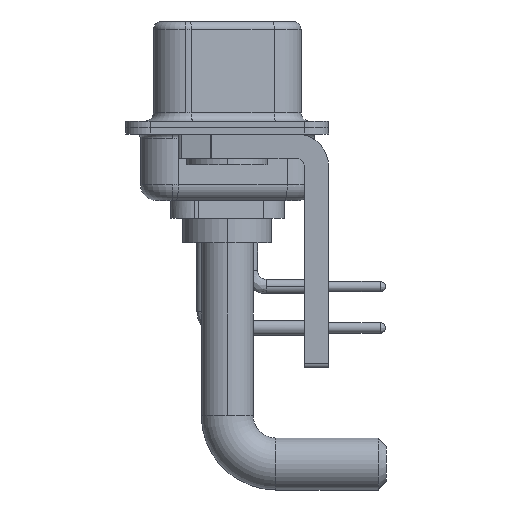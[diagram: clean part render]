
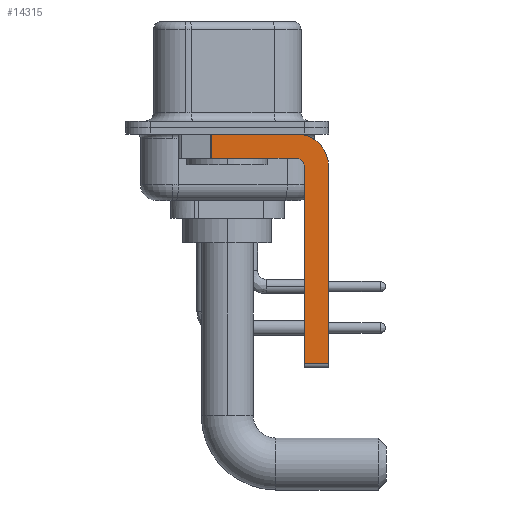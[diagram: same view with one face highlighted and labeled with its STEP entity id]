
A CAD part, left-side view. The second image highlights one B-rep face of the part: STEP entity #14315.
In plain terms, the highlighted planar face has unit normal (-1, 0, 0).
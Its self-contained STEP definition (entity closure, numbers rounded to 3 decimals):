
#179 = VERTEX_POINT ( 'NONE', #17089 ) ;
#199 = CARTESIAN_POINT ( 'NONE',  ( -2.9, -6.25, -2.4 ) ) ;
#289 = PLANE ( 'NONE',  #7650 ) ;
#544 = DIRECTION ( 'NONE',  ( 1., 0., 0. ) ) ;
#666 = DIRECTION ( 'NONE',  ( 0., 0., -1. ) ) ;
#1107 = ORIENTED_EDGE ( 'NONE', *, *, #8212, .T. ) ;
#1223 = ORIENTED_EDGE ( 'NONE', *, *, #15616, .F. ) ;
#1299 = CARTESIAN_POINT ( 'NONE',  ( -2.9, -4.25, -0.4 ) ) ;
#1308 = ORIENTED_EDGE ( 'NONE', *, *, #18619, .F. ) ;
#1354 = VERTEX_POINT ( 'NONE', #23526 ) ;
#1426 = CARTESIAN_POINT ( 'NONE',  ( -2.9, -4.75, -14.8 ) ) ;
#1661 = LINE ( 'NONE', #19299, #11949 ) ;
#1909 = VECTOR ( 'NONE', #19220, 1000. ) ;
#2603 = LINE ( 'NONE', #199, #24019 ) ;
#2900 = VERTEX_POINT ( 'NONE', #15469 ) ;
#3135 = DIRECTION ( 'NONE',  ( 0., 0., 1. ) ) ;
#3473 = CARTESIAN_POINT ( 'NONE',  ( -2.9, -4.75, -2.4 ) ) ;
#3870 = LINE ( 'NONE', #11405, #1909 ) ;
#4006 = EDGE_CURVE ( 'NONE', #9132, #5978, #2603, .T. ) ;
#4543 = ORIENTED_EDGE ( 'NONE', *, *, #11227, .F. ) ;
#5122 = LINE ( 'NONE', #24439, #6893 ) ;
#5454 = CARTESIAN_POINT ( 'NONE',  ( -2.9, -4.25, -1.9 ) ) ;
#5978 = VERTEX_POINT ( 'NONE', #25233 ) ;
#6893 = VECTOR ( 'NONE', #12913, 1000. ) ;
#7650 = AXIS2_PLACEMENT_3D ( 'NONE', #21753, #544, #666 ) ;
#8212 = EDGE_CURVE ( 'NONE', #1354, #5978, #1661, .T. ) ;
#8398 = ORIENTED_EDGE ( 'NONE', *, *, #4006, .F. ) ;
#9132 = VERTEX_POINT ( 'NONE', #16945 ) ;
#9270 = DIRECTION ( 'NONE',  ( 0., 0., -1. ) ) ;
#9562 = LINE ( 'NONE', #13260, #20406 ) ;
#9679 = DIRECTION ( 'NONE',  ( 0., 1., 0. ) ) ;
#9888 = VERTEX_POINT ( 'NONE', #5454 ) ;
#10363 = ORIENTED_EDGE ( 'NONE', *, *, #16219, .F. ) ;
#11005 = DIRECTION ( 'NONE',  ( 0., 0., 1. ) ) ;
#11227 = EDGE_CURVE ( 'NONE', #1354, #20185, #12912, .T. ) ;
#11405 = CARTESIAN_POINT ( 'NONE',  ( -2.9, 0.978, -1.9 ) ) ;
#11949 = VECTOR ( 'NONE', #25048, 1000. ) ;
#12036 = DIRECTION ( 'NONE',  ( 0., 0., -1. ) ) ;
#12064 = EDGE_CURVE ( 'NONE', #2900, #179, #3870, .T. ) ;
#12137 = FACE_OUTER_BOUND ( 'NONE', #15425, .T. ) ;
#12811 = VECTOR ( 'NONE', #11005, 1000. ) ;
#12912 = LINE ( 'NONE', #1426, #12811 ) ;
#12913 = DIRECTION ( 'NONE',  ( 0., -1., 0. ) ) ;
#13260 = CARTESIAN_POINT ( 'NONE',  ( -2.9, -4.25, -1.9 ) ) ;
#13633 = EDGE_CURVE ( 'NONE', #24718, #9132, #19455, .T. ) ;
#14315 = ADVANCED_FACE ( 'NONE', ( #12137 ), #289, .F. ) ;
#14343 = CIRCLE ( 'NONE', #19671, 0.5 ) ;
#15425 = EDGE_LOOP ( 'NONE', ( #1223, #15513, #10363, #1308, #4543, #1107, #8398, #17391 ) ) ;
#15429 = AXIS2_PLACEMENT_3D ( 'NONE', #22838, #24877, #9270 ) ;
#15469 = CARTESIAN_POINT ( 'NONE',  ( -2.9, 0.978, -0.4 ) ) ;
#15513 = ORIENTED_EDGE ( 'NONE', *, *, #12064, .T. ) ;
#15616 = EDGE_CURVE ( 'NONE', #2900, #24718, #5122, .T. ) ;
#16219 = EDGE_CURVE ( 'NONE', #9888, #179, #9562, .T. ) ;
#16945 = CARTESIAN_POINT ( 'NONE',  ( -2.9, -6.25, -2.4 ) ) ;
#17089 = CARTESIAN_POINT ( 'NONE',  ( -2.9, 0.978, -1.9 ) ) ;
#17391 = ORIENTED_EDGE ( 'NONE', *, *, #13633, .F. ) ;
#18619 = EDGE_CURVE ( 'NONE', #20185, #9888, #14343, .T. ) ;
#19220 = DIRECTION ( 'NONE',  ( 0., 0., -1. ) ) ;
#19299 = CARTESIAN_POINT ( 'NONE',  ( -2.9, -4.25, -14.55 ) ) ;
#19455 = CIRCLE ( 'NONE', #15429, 2. ) ;
#19671 = AXIS2_PLACEMENT_3D ( 'NONE', #24987, #20652, #3135 ) ;
#20185 = VERTEX_POINT ( 'NONE', #3473 ) ;
#20406 = VECTOR ( 'NONE', #9679, 1000. ) ;
#20652 = DIRECTION ( 'NONE',  ( -1., 0., 0. ) ) ;
#21753 = CARTESIAN_POINT ( 'NONE',  ( -2.9, -4.25, -2.4 ) ) ;
#22838 = CARTESIAN_POINT ( 'NONE',  ( -2.9, -4.25, -2.4 ) ) ;
#23526 = CARTESIAN_POINT ( 'NONE',  ( -2.9, -4.75, -14.55 ) ) ;
#24019 = VECTOR ( 'NONE', #12036, 1000. ) ;
#24439 = CARTESIAN_POINT ( 'NONE',  ( -2.9, 3., -0.4 ) ) ;
#24718 = VERTEX_POINT ( 'NONE', #1299 ) ;
#24877 = DIRECTION ( 'NONE',  ( 1., 0., 0. ) ) ;
#24987 = CARTESIAN_POINT ( 'NONE',  ( -2.9, -4.25, -2.4 ) ) ;
#25048 = DIRECTION ( 'NONE',  ( 0., -1., 0. ) ) ;
#25233 = CARTESIAN_POINT ( 'NONE',  ( -2.9, -6.25, -14.55 ) ) ;
